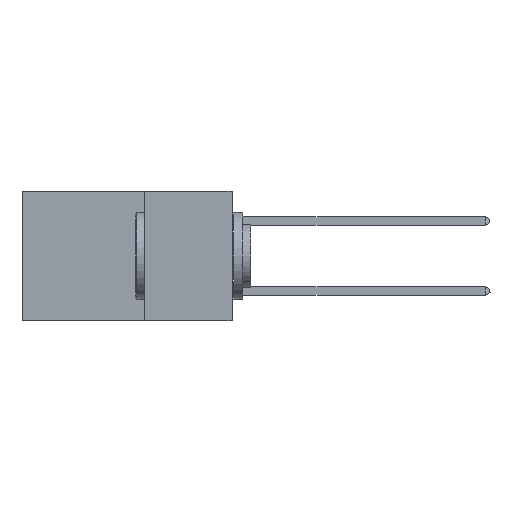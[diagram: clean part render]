
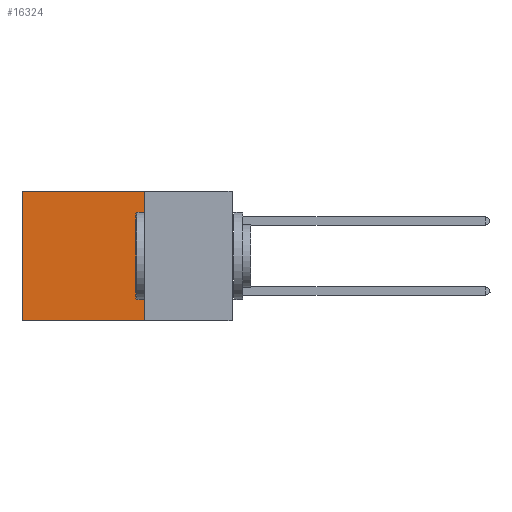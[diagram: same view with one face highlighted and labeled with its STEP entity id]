
A CAD part, left-side view. The second image highlights one B-rep face of the part: STEP entity #16324.
In plain terms, the highlighted planar face has unit normal (-1, 0, 0).
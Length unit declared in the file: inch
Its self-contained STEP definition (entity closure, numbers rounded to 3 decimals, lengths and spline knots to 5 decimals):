
#75 = CARTESIAN_POINT ( 'NONE',  ( 0.2875, 0.25, -0.37 ) ) ;
#287 = VERTEX_POINT ( 'NONE', #19766 ) ;
#461 = VECTOR ( 'NONE', #25858, 39.37008 ) ;
#2151 = VECTOR ( 'NONE', #32873, 39.37008 ) ;
#3685 = VERTEX_POINT ( 'NONE', #9387 ) ;
#4712 = FACE_OUTER_BOUND ( 'NONE', #29193, .T. ) ;
#5734 = DIRECTION ( 'NONE',  ( 1., 0., 0. ) ) ;
#6357 = ORIENTED_EDGE ( 'NONE', *, *, #19236, .F. ) ;
#6526 = EDGE_CURVE ( 'NONE', #31730, #25515, #18863, .T. ) ;
#7134 = AXIS2_PLACEMENT_3D ( 'NONE', #29380, #5734, #31782 ) ;
#7390 = CARTESIAN_POINT ( 'NONE',  ( 0.2875, 0.6, 0. ) ) ;
#8539 = DIRECTION ( 'NONE',  ( 0., 0., -1. ) ) ;
#9387 = CARTESIAN_POINT ( 'NONE',  ( 0.2875, 0.6, -0.37 ) ) ;
#11037 = LINE ( 'NONE', #7390, #21548 ) ;
#11400 = EDGE_CURVE ( 'NONE', #287, #3685, #11037, .T. ) ;
#11476 = ORIENTED_EDGE ( 'NONE', *, *, #14299, .T. ) ;
#12815 = CARTESIAN_POINT ( 'NONE',  ( 0.2875, 0.25, -0.37 ) ) ;
#14299 = EDGE_CURVE ( 'NONE', #31730, #287, #16601, .T. ) ;
#14571 = CARTESIAN_POINT ( 'NONE',  ( 0.2875, 0.25, 0. ) ) ;
#15337 = PLANE ( 'NONE',  #7134 ) ;
#16324 = ADVANCED_FACE ( 'NONE', ( #4712 ), #15337, .F. ) ;
#16601 = LINE ( 'NONE', #14571, #2151 ) ;
#18863 = LINE ( 'NONE', #26821, #20077 ) ;
#19236 = EDGE_CURVE ( 'NONE', #25515, #3685, #19932, .T. ) ;
#19766 = CARTESIAN_POINT ( 'NONE',  ( 0.2875, 0.6, 0. ) ) ;
#19932 = LINE ( 'NONE', #12815, #461 ) ;
#20077 = VECTOR ( 'NONE', #8539, 39.37008 ) ;
#21548 = VECTOR ( 'NONE', #30473, 39.37008 ) ;
#23970 = ORIENTED_EDGE ( 'NONE', *, *, #6526, .F. ) ;
#25515 = VERTEX_POINT ( 'NONE', #75 ) ;
#25858 = DIRECTION ( 'NONE',  ( 0., 1., 0. ) ) ;
#26024 = CARTESIAN_POINT ( 'NONE',  ( 0.2875, 0.25, 0. ) ) ;
#26821 = CARTESIAN_POINT ( 'NONE',  ( 0.2875, 0.25, 0. ) ) ;
#28095 = ORIENTED_EDGE ( 'NONE', *, *, #11400, .T. ) ;
#29193 = EDGE_LOOP ( 'NONE', ( #28095, #6357, #23970, #11476 ) ) ;
#29380 = CARTESIAN_POINT ( 'NONE',  ( 0.2875, 0.25, 0. ) ) ;
#30473 = DIRECTION ( 'NONE',  ( 0., 0., -1. ) ) ;
#31730 = VERTEX_POINT ( 'NONE', #26024 ) ;
#31782 = DIRECTION ( 'NONE',  ( 0., 0., -1. ) ) ;
#32873 = DIRECTION ( 'NONE',  ( 0., 1., 0. ) ) ;
